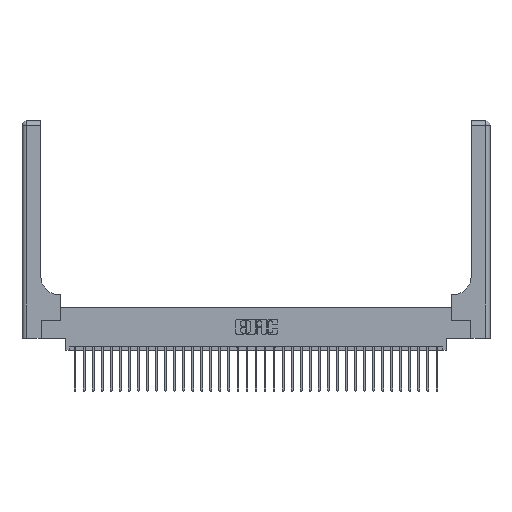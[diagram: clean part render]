
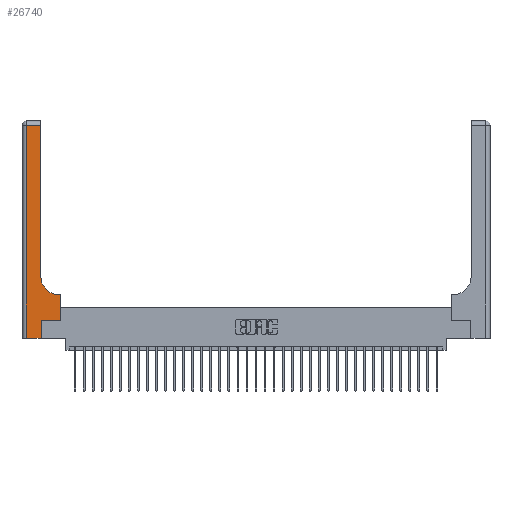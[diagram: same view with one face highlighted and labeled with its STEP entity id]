
A CAD part, top view. The second image highlights one B-rep face of the part: STEP entity #26740.
In plain terms, the highlighted planar face has unit normal (0, 0, 1).
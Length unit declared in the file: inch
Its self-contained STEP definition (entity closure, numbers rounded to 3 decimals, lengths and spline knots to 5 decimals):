
#154 = CARTESIAN_POINT ( 'NONE',  ( 0.26, 3., 0.37 ) ) ;
#1098 = EDGE_LOOP ( 'NONE', ( #11579, #27211, #6352, #21095, #22550, #2304, #2865, #24503, #21244 ) ) ;
#2152 = CARTESIAN_POINT ( 'NONE',  ( 0.51, 0.85, 0.37 ) ) ;
#2304 = ORIENTED_EDGE ( 'NONE', *, *, #27633, .T. ) ;
#2373 = VERTEX_POINT ( 'NONE', #30193 ) ;
#2688 = LINE ( 'NONE', #154, #26343 ) ;
#2865 = ORIENTED_EDGE ( 'NONE', *, *, #10475, .T. ) ;
#3008 = FACE_OUTER_BOUND ( 'NONE', #1098, .T. ) ;
#3859 = VERTEX_POINT ( 'NONE', #27245 ) ;
#4800 = DIRECTION ( 'NONE',  ( 0., 0., -1. ) ) ;
#5106 = VERTEX_POINT ( 'NONE', #6893 ) ;
#5175 = PLANE ( 'NONE',  #9293 ) ;
#5482 = VECTOR ( 'NONE', #5518, 39.37008 ) ;
#5518 = DIRECTION ( 'NONE',  ( 0., 1., 0. ) ) ;
#5679 = LINE ( 'NONE', #8501, #23981 ) ;
#6352 = ORIENTED_EDGE ( 'NONE', *, *, #28764, .T. ) ;
#6442 = DIRECTION ( 'NONE',  ( 1., 0., 0. ) ) ;
#6893 = CARTESIAN_POINT ( 'NONE',  ( 0.528, 0.6, 0.37 ) ) ;
#7658 = VECTOR ( 'NONE', #24461, 39.37008 ) ;
#8501 = CARTESIAN_POINT ( 'NONE',  ( 0., 0., 0.37 ) ) ;
#8859 = LINE ( 'NONE', #27035, #21877 ) ;
#8987 = EDGE_CURVE ( 'NONE', #5106, #19617, #8859, .T. ) ;
#9025 = EDGE_CURVE ( 'NONE', #29243, #28175, #24878, .T. ) ;
#9293 = AXIS2_PLACEMENT_3D ( 'NONE', #15284, #25691, #22868 ) ;
#9737 = CARTESIAN_POINT ( 'NONE',  ( 0.06, 3., 0.37 ) ) ;
#9843 = CARTESIAN_POINT ( 'NONE',  ( 0., 2.94, 0.37 ) ) ;
#10452 = EDGE_CURVE ( 'NONE', #21086, #13621, #5679, .T. ) ;
#10475 = EDGE_CURVE ( 'NONE', #12577, #5106, #28689, .T. ) ;
#10672 = VECTOR ( 'NONE', #22520, 39.37008 ) ;
#10892 = CARTESIAN_POINT ( 'NONE',  ( 0.26, 2.94, 0.37 ) ) ;
#11579 = ORIENTED_EDGE ( 'NONE', *, *, #32584, .T. ) ;
#11958 = VECTOR ( 'NONE', #6442, 39.37008 ) ;
#12577 = VERTEX_POINT ( 'NONE', #26606 ) ;
#13441 = EDGE_CURVE ( 'NONE', #19617, #3859, #32644, .T. ) ;
#13621 = VERTEX_POINT ( 'NONE', #28289 ) ;
#14967 = CARTESIAN_POINT ( 'NONE',  ( 0.06, 2.94, 0.37 ) ) ;
#15284 = CARTESIAN_POINT ( 'NONE',  ( 0., 3., 0.37 ) ) ;
#16467 = DIRECTION ( 'NONE',  ( -1., 0., 0. ) ) ;
#18089 = CARTESIAN_POINT ( 'NONE',  ( 0.528, 0.25, 0.37 ) ) ;
#18280 = EDGE_CURVE ( 'NONE', #13621, #2373, #22189, .T. ) ;
#19377 = CARTESIAN_POINT ( 'NONE',  ( 0.265, 0., 0.37 ) ) ;
#19617 = VERTEX_POINT ( 'NONE', #21089 ) ;
#19913 = DIRECTION ( 'NONE',  ( -1., 0., 0. ) ) ;
#20735 = DIRECTION ( 'NONE',  ( 1., 0., 0. ) ) ;
#21086 = VERTEX_POINT ( 'NONE', #28190 ) ;
#21089 = CARTESIAN_POINT ( 'NONE',  ( 0.51, 0.6, 0.37 ) ) ;
#21095 = ORIENTED_EDGE ( 'NONE', *, *, #10452, .T. ) ;
#21244 = ORIENTED_EDGE ( 'NONE', *, *, #13441, .T. ) ;
#21877 = VECTOR ( 'NONE', #16467, 39.37008 ) ;
#22189 = LINE ( 'NONE', #19377, #10672 ) ;
#22520 = DIRECTION ( 'NONE',  ( 0., 1., 0. ) ) ;
#22550 = ORIENTED_EDGE ( 'NONE', *, *, #18280, .T. ) ;
#22868 = DIRECTION ( 'NONE',  ( -1., 0., 0. ) ) ;
#23981 = VECTOR ( 'NONE', #20735, 39.37008 ) ;
#24461 = DIRECTION ( 'NONE',  ( 0., -1., 0. ) ) ;
#24503 = ORIENTED_EDGE ( 'NONE', *, *, #8987, .T. ) ;
#24878 = LINE ( 'NONE', #9843, #31430 ) ;
#25307 = DIRECTION ( 'NONE',  ( 0., 1., 0. ) ) ;
#25691 = DIRECTION ( 'NONE',  ( 0., 0., -1. ) ) ;
#26343 = VECTOR ( 'NONE', #25307, 39.37008 ) ;
#26606 = CARTESIAN_POINT ( 'NONE',  ( 0.528, 0.25, 0.37 ) ) ;
#26740 = ADVANCED_FACE ( 'NONE', ( #3008 ), #5175, .F. ) ;
#27035 = CARTESIAN_POINT ( 'NONE',  ( 0.26, 0.6, 0.37 ) ) ;
#27141 = DIRECTION ( 'NONE',  ( 1., 0., 0. ) ) ;
#27211 = ORIENTED_EDGE ( 'NONE', *, *, #9025, .T. ) ;
#27245 = CARTESIAN_POINT ( 'NONE',  ( 0.26, 0.85, 0.37 ) ) ;
#27633 = EDGE_CURVE ( 'NONE', #2373, #12577, #30219, .T. ) ;
#28175 = VERTEX_POINT ( 'NONE', #14967 ) ;
#28190 = CARTESIAN_POINT ( 'NONE',  ( 0.06, 0., 0.37 ) ) ;
#28289 = CARTESIAN_POINT ( 'NONE',  ( 0.265, 0., 0.37 ) ) ;
#28689 = LINE ( 'NONE', #18089, #5482 ) ;
#28764 = EDGE_CURVE ( 'NONE', #28175, #21086, #32392, .T. ) ;
#29115 = CARTESIAN_POINT ( 'NONE',  ( 0.265, 0.25, 0.37 ) ) ;
#29243 = VERTEX_POINT ( 'NONE', #10892 ) ;
#30193 = CARTESIAN_POINT ( 'NONE',  ( 0.265, 0.25, 0.37 ) ) ;
#30219 = LINE ( 'NONE', #29115, #11958 ) ;
#31430 = VECTOR ( 'NONE', #19913, 39.37008 ) ;
#31598 = AXIS2_PLACEMENT_3D ( 'NONE', #2152, #4800, #27141 ) ;
#32392 = LINE ( 'NONE', #9737, #7658 ) ;
#32584 = EDGE_CURVE ( 'NONE', #3859, #29243, #2688, .T. ) ;
#32644 = CIRCLE ( 'NONE', #31598, 0.25 ) ;
